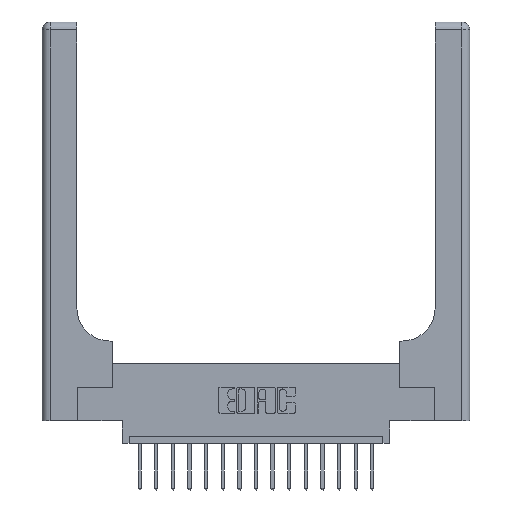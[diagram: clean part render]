
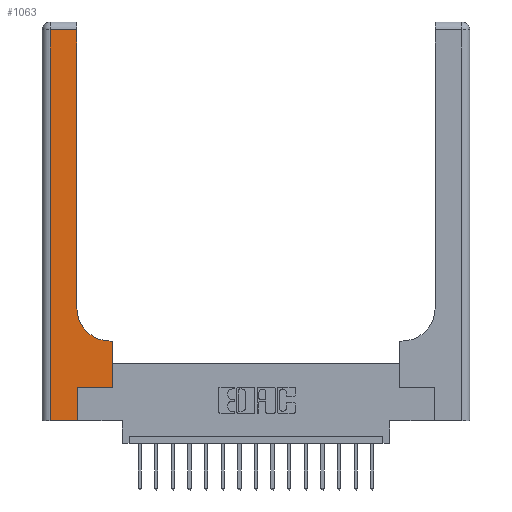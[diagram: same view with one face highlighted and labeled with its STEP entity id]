
A CAD part, top view. The second image highlights one B-rep face of the part: STEP entity #1063.
In plain terms, the highlighted planar face has unit normal (0, 0, 1).
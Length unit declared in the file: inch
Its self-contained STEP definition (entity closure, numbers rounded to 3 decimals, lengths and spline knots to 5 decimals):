
#60 = EDGE_LOOP ( 'NONE', ( #3998, #8887, #16550, #10034, #10231, #6011, #17083, #14499, #13709 ) ) ;
#267 = CARTESIAN_POINT ( 'NONE',  ( 0.06, 3., 0.37 ) ) ;
#634 = VECTOR ( 'NONE', #980, 39.37008 ) ;
#690 = VECTOR ( 'NONE', #13084, 39.37008 ) ;
#941 = AXIS2_PLACEMENT_3D ( 'NONE', #9958, #15672, #12798 ) ;
#980 = DIRECTION ( 'NONE',  ( 0., 1., 0. ) ) ;
#1063 = ADVANCED_FACE ( 'NONE', ( #9330 ), #17760, .F. ) ;
#1253 = EDGE_CURVE ( 'NONE', #14166, #7398, #7778, .T. ) ;
#1590 = VECTOR ( 'NONE', #5426, 39.37008 ) ;
#2034 = AXIS2_PLACEMENT_3D ( 'NONE', #16112, #10887, #11586 ) ;
#2164 = CARTESIAN_POINT ( 'NONE',  ( 0.528, 0.25, 0.37 ) ) ;
#2302 = DIRECTION ( 'NONE',  ( -1., 0., 0. ) ) ;
#3100 = CARTESIAN_POINT ( 'NONE',  ( 0.265, 0.25, 0.37 ) ) ;
#3422 = EDGE_CURVE ( 'NONE', #7398, #15886, #4364, .T. ) ;
#3927 = CIRCLE ( 'NONE', #941, 0.25 ) ;
#3998 = ORIENTED_EDGE ( 'NONE', *, *, #11490, .T. ) ;
#4364 = LINE ( 'NONE', #16262, #634 ) ;
#4503 = CARTESIAN_POINT ( 'NONE',  ( 0.06, 0., 0.37 ) ) ;
#4605 = EDGE_CURVE ( 'NONE', #11846, #5520, #6661, .T. ) ;
#5060 = CARTESIAN_POINT ( 'NONE',  ( 0.528, 0.6, 0.37 ) ) ;
#5426 = DIRECTION ( 'NONE',  ( -1., 0., 0. ) ) ;
#5520 = VERTEX_POINT ( 'NONE', #12355 ) ;
#5537 = DIRECTION ( 'NONE',  ( 0., 1., 0. ) ) ;
#6011 = ORIENTED_EDGE ( 'NONE', *, *, #1253, .T. ) ;
#6216 = VECTOR ( 'NONE', #2302, 39.37008 ) ;
#6360 = CARTESIAN_POINT ( 'NONE',  ( 0., 2.94, 0.37 ) ) ;
#6661 = LINE ( 'NONE', #6360, #6216 ) ;
#6838 = CARTESIAN_POINT ( 'NONE',  ( 0.265, 0., 0.37 ) ) ;
#7180 = VECTOR ( 'NONE', #18089, 39.37008 ) ;
#7398 = VERTEX_POINT ( 'NONE', #2164 ) ;
#7654 = LINE ( 'NONE', #6838, #14760 ) ;
#7778 = LINE ( 'NONE', #16114, #10867 ) ;
#8098 = EDGE_CURVE ( 'NONE', #14711, #14166, #7654, .T. ) ;
#8155 = EDGE_CURVE ( 'NONE', #17606, #12558, #3927, .T. ) ;
#8887 = ORIENTED_EDGE ( 'NONE', *, *, #4605, .T. ) ;
#9330 = FACE_OUTER_BOUND ( 'NONE', #60, .T. ) ;
#9504 = CARTESIAN_POINT ( 'NONE',  ( 0.265, 0., 0.37 ) ) ;
#9958 = CARTESIAN_POINT ( 'NONE',  ( 0.51, 0.85, 0.37 ) ) ;
#10034 = ORIENTED_EDGE ( 'NONE', *, *, #15937, .T. ) ;
#10231 = ORIENTED_EDGE ( 'NONE', *, *, #8098, .T. ) ;
#10252 = LINE ( 'NONE', #17481, #7180 ) ;
#10412 = LINE ( 'NONE', #14713, #13511 ) ;
#10463 = CARTESIAN_POINT ( 'NONE',  ( 0.51, 0.6, 0.37 ) ) ;
#10867 = VECTOR ( 'NONE', #14529, 39.37008 ) ;
#10887 = DIRECTION ( 'NONE',  ( 0., 0., -1. ) ) ;
#11490 = EDGE_CURVE ( 'NONE', #12558, #11846, #10412, .T. ) ;
#11500 = CARTESIAN_POINT ( 'NONE',  ( 0.26, 2.94, 0.37 ) ) ;
#11586 = DIRECTION ( 'NONE',  ( -1., 0., 0. ) ) ;
#11846 = VERTEX_POINT ( 'NONE', #11500 ) ;
#12106 = VERTEX_POINT ( 'NONE', #4503 ) ;
#12355 = CARTESIAN_POINT ( 'NONE',  ( 0.06, 2.94, 0.37 ) ) ;
#12558 = VERTEX_POINT ( 'NONE', #13014 ) ;
#12798 = DIRECTION ( 'NONE',  ( 1., 0., 0. ) ) ;
#12938 = EDGE_CURVE ( 'NONE', #5520, #12106, #17700, .T. ) ;
#12989 = EDGE_CURVE ( 'NONE', #15886, #17606, #15046, .T. ) ;
#13014 = CARTESIAN_POINT ( 'NONE',  ( 0.26, 0.85, 0.37 ) ) ;
#13084 = DIRECTION ( 'NONE',  ( 0., -1., 0. ) ) ;
#13511 = VECTOR ( 'NONE', #17288, 39.37008 ) ;
#13709 = ORIENTED_EDGE ( 'NONE', *, *, #8155, .T. ) ;
#13840 = CARTESIAN_POINT ( 'NONE',  ( 0.26, 0.6, 0.37 ) ) ;
#14166 = VERTEX_POINT ( 'NONE', #3100 ) ;
#14499 = ORIENTED_EDGE ( 'NONE', *, *, #12989, .T. ) ;
#14529 = DIRECTION ( 'NONE',  ( 1., 0., 0. ) ) ;
#14711 = VERTEX_POINT ( 'NONE', #9504 ) ;
#14713 = CARTESIAN_POINT ( 'NONE',  ( 0.26, 3., 0.37 ) ) ;
#14760 = VECTOR ( 'NONE', #5537, 39.37008 ) ;
#15046 = LINE ( 'NONE', #13840, #1590 ) ;
#15672 = DIRECTION ( 'NONE',  ( 0., 0., -1. ) ) ;
#15886 = VERTEX_POINT ( 'NONE', #5060 ) ;
#15937 = EDGE_CURVE ( 'NONE', #12106, #14711, #10252, .T. ) ;
#16112 = CARTESIAN_POINT ( 'NONE',  ( 0., 3., 0.37 ) ) ;
#16114 = CARTESIAN_POINT ( 'NONE',  ( 0.265, 0.25, 0.37 ) ) ;
#16262 = CARTESIAN_POINT ( 'NONE',  ( 0.528, 0.25, 0.37 ) ) ;
#16550 = ORIENTED_EDGE ( 'NONE', *, *, #12938, .T. ) ;
#17083 = ORIENTED_EDGE ( 'NONE', *, *, #3422, .T. ) ;
#17288 = DIRECTION ( 'NONE',  ( 0., 1., 0. ) ) ;
#17481 = CARTESIAN_POINT ( 'NONE',  ( 0., 0., 0.37 ) ) ;
#17606 = VERTEX_POINT ( 'NONE', #10463 ) ;
#17700 = LINE ( 'NONE', #267, #690 ) ;
#17760 = PLANE ( 'NONE',  #2034 ) ;
#18089 = DIRECTION ( 'NONE',  ( 1., 0., 0. ) ) ;
